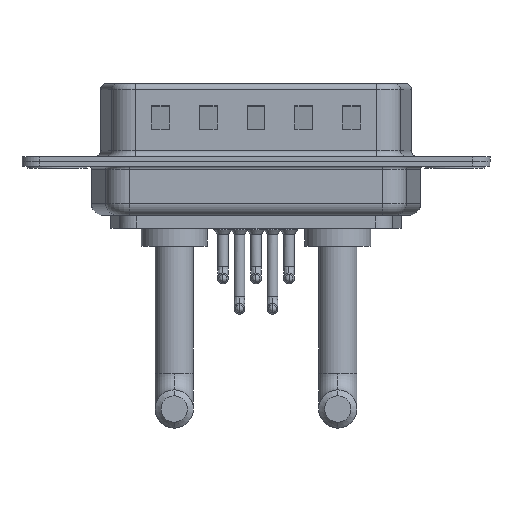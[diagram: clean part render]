
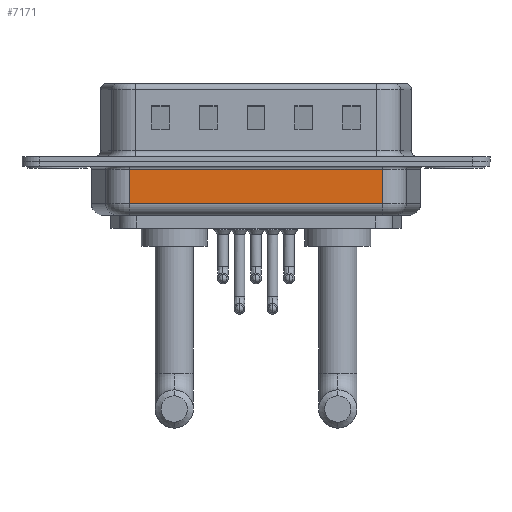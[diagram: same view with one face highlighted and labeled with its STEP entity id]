
A CAD part, front view. The second image highlights one B-rep face of the part: STEP entity #7171.
In plain terms, the highlighted planar face has unit normal (0, -1, 0).
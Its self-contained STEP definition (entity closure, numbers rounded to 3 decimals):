
#67 = LINE ( 'NONE', #7135, #13724 ) ;
#559 = ORIENTED_EDGE ( 'NONE', *, *, #10589, .F. ) ;
#1345 = FACE_OUTER_BOUND ( 'NONE', #15907, .T. ) ;
#1891 = AXIS2_PLACEMENT_3D ( 'NONE', #14309, #7337, #11302 ) ;
#2147 = CARTESIAN_POINT ( 'NONE',  ( 6.031, -5.35, -0.65 ) ) ;
#2592 = ORIENTED_EDGE ( 'NONE', *, *, #4703, .T. ) ;
#3169 = DIRECTION ( 'NONE',  ( 0., 0., 1. ) ) ;
#3334 = VECTOR ( 'NONE', #3169, 1000. ) ;
#3481 = ORIENTED_EDGE ( 'NONE', *, *, #14207, .T. ) ;
#3500 = LINE ( 'NONE', #2147, #7645 ) ;
#4634 = ORIENTED_EDGE ( 'NONE', *, *, #7498, .T. ) ;
#4703 = EDGE_CURVE ( 'NONE', #8361, #11491, #3500, .T. ) ;
#5041 = DIRECTION ( 'NONE',  ( -1., 0., 0. ) ) ;
#5296 = VECTOR ( 'NONE', #11100, 1000. ) ;
#5497 = VERTEX_POINT ( 'NONE', #18793 ) ;
#7135 = CARTESIAN_POINT ( 'NONE',  ( 6.031, -5.35, -4.5 ) ) ;
#7171 = ADVANCED_FACE ( 'NONE', ( #1345 ), #16146, .F. ) ;
#7337 = DIRECTION ( 'NONE',  ( 0., 1., 0. ) ) ;
#7498 = EDGE_CURVE ( 'NONE', #5497, #9690, #9728, .T. ) ;
#7645 = VECTOR ( 'NONE', #5041, 1000. ) ;
#8361 = VERTEX_POINT ( 'NONE', #14024 ) ;
#9690 = VERTEX_POINT ( 'NONE', #17625 ) ;
#9728 = LINE ( 'NONE', #15465, #5296 ) ;
#10506 = LINE ( 'NONE', #16422, #3334 ) ;
#10589 = EDGE_CURVE ( 'NONE', #5497, #11491, #67, .T. ) ;
#11100 = DIRECTION ( 'NONE',  ( 1., 0., 0. ) ) ;
#11302 = DIRECTION ( 'NONE',  ( 0., 0., 1. ) ) ;
#11491 = VERTEX_POINT ( 'NONE', #13705 ) ;
#13705 = CARTESIAN_POINT ( 'NONE',  ( 6.031, -5.35, -0.65 ) ) ;
#13724 = VECTOR ( 'NONE', #14766, 1000. ) ;
#14024 = CARTESIAN_POINT ( 'NONE',  ( 27.269, -5.35, -0.65 ) ) ;
#14207 = EDGE_CURVE ( 'NONE', #9690, #8361, #10506, .T. ) ;
#14309 = CARTESIAN_POINT ( 'NONE',  ( 6.031, -5.35, -4.5 ) ) ;
#14766 = DIRECTION ( 'NONE',  ( 0., 0., 1. ) ) ;
#15465 = CARTESIAN_POINT ( 'NONE',  ( 6.031, -5.35, -3.5 ) ) ;
#15907 = EDGE_LOOP ( 'NONE', ( #559, #4634, #3481, #2592 ) ) ;
#16146 = PLANE ( 'NONE',  #1891 ) ;
#16422 = CARTESIAN_POINT ( 'NONE',  ( 27.269, -5.35, -4.5 ) ) ;
#17625 = CARTESIAN_POINT ( 'NONE',  ( 27.269, -5.35, -3.5 ) ) ;
#18793 = CARTESIAN_POINT ( 'NONE',  ( 6.031, -5.35, -3.5 ) ) ;
